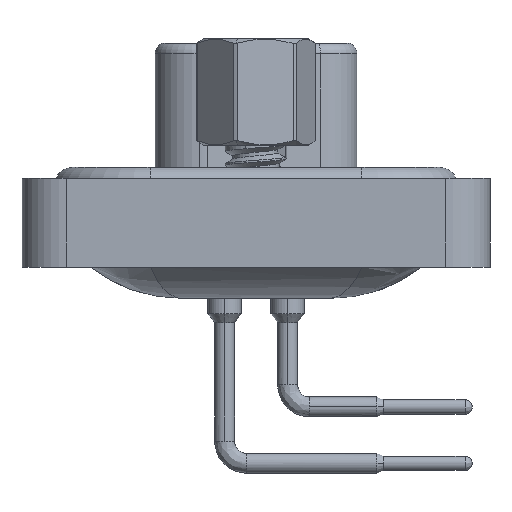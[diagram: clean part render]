
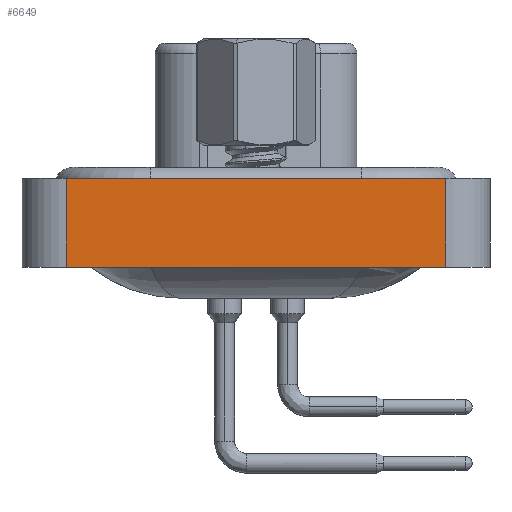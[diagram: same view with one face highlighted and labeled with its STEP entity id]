
A CAD part, left-side view. The second image highlights one B-rep face of the part: STEP entity #6649.
In plain terms, the highlighted planar face has unit normal (-1, 0, 0).
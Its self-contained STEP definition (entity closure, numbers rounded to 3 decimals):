
#755 = CARTESIAN_POINT ( 'NONE',  ( -7.26, -8.55, 0.4 ) ) ;
#1003 = VERTEX_POINT ( 'NONE', #22382 ) ;
#1046 = CARTESIAN_POINT ( 'NONE',  ( -7.26, 8.55, -3.6 ) ) ;
#1391 = PLANE ( 'NONE',  #18347 ) ;
#2920 = EDGE_LOOP ( 'NONE', ( #11656, #3872, #23089, #6078 ) ) ;
#3872 = ORIENTED_EDGE ( 'NONE', *, *, #13919, .F. ) ;
#4176 = CARTESIAN_POINT ( 'NONE',  ( -7.26, -8.55, 0.4 ) ) ;
#4773 = VECTOR ( 'NONE', #15151, 1000. ) ;
#5458 = CARTESIAN_POINT ( 'NONE',  ( -7.26, -8.55, -3.6 ) ) ;
#5909 = VERTEX_POINT ( 'NONE', #24803 ) ;
#6078 = ORIENTED_EDGE ( 'NONE', *, *, #10385, .T. ) ;
#6649 = ADVANCED_FACE ( 'NONE', ( #17198 ), #1391, .T. ) ;
#6915 = LINE ( 'NONE', #14719, #18135 ) ;
#7191 = VECTOR ( 'NONE', #10683, 1000. ) ;
#8047 = EDGE_CURVE ( 'NONE', #17252, #1003, #18257, .T. ) ;
#8704 = DIRECTION ( 'NONE',  ( 0., -1., 0. ) ) ;
#8807 = DIRECTION ( 'NONE',  ( 0., 0., 1. ) ) ;
#8879 = CARTESIAN_POINT ( 'NONE',  ( -7.26, -8.55, -3.6 ) ) ;
#10385 = EDGE_CURVE ( 'NONE', #17252, #5909, #6915, .T. ) ;
#10683 = DIRECTION ( 'NONE',  ( 0., -1., 0. ) ) ;
#10927 = LINE ( 'NONE', #755, #7191 ) ;
#11085 = VECTOR ( 'NONE', #8807, 1000. ) ;
#11656 = ORIENTED_EDGE ( 'NONE', *, *, #24496, .T. ) ;
#13234 = CARTESIAN_POINT ( 'NONE',  ( -7.26, 8.55, -3.6 ) ) ;
#13919 = EDGE_CURVE ( 'NONE', #1003, #24780, #10927, .T. ) ;
#14719 = CARTESIAN_POINT ( 'NONE',  ( -7.26, -8.55, -3.6 ) ) ;
#14781 = LINE ( 'NONE', #8879, #4773 ) ;
#15151 = DIRECTION ( 'NONE',  ( 0., 0., 1. ) ) ;
#17198 = FACE_OUTER_BOUND ( 'NONE', #2920, .T. ) ;
#17252 = VERTEX_POINT ( 'NONE', #13234 ) ;
#18135 = VECTOR ( 'NONE', #8704, 1000. ) ;
#18257 = LINE ( 'NONE', #1046, #11085 ) ;
#18347 = AXIS2_PLACEMENT_3D ( 'NONE', #5458, #24689, #20886 ) ;
#20886 = DIRECTION ( 'NONE',  ( 0., 0., 1. ) ) ;
#22382 = CARTESIAN_POINT ( 'NONE',  ( -7.26, 8.55, 0.4 ) ) ;
#23089 = ORIENTED_EDGE ( 'NONE', *, *, #8047, .F. ) ;
#24496 = EDGE_CURVE ( 'NONE', #5909, #24780, #14781, .T. ) ;
#24689 = DIRECTION ( 'NONE',  ( -1., 0., 0. ) ) ;
#24780 = VERTEX_POINT ( 'NONE', #4176 ) ;
#24803 = CARTESIAN_POINT ( 'NONE',  ( -7.26, -8.55, -3.6 ) ) ;
